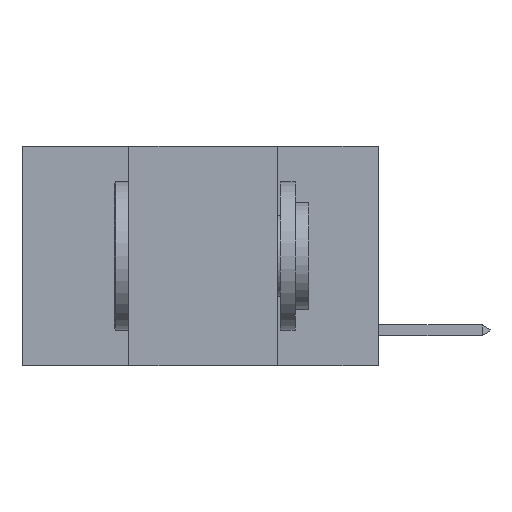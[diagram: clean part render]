
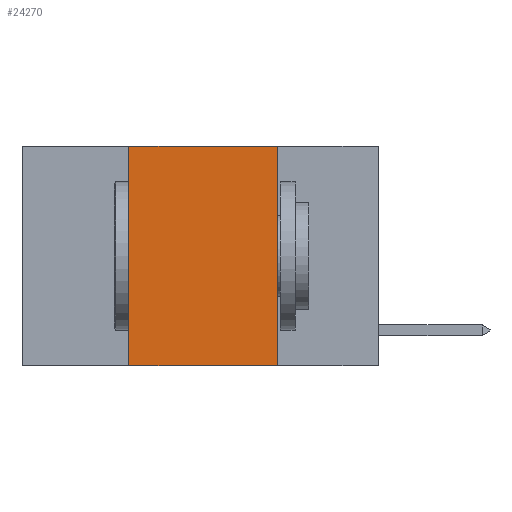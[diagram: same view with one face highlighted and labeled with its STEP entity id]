
A CAD part, left-side view. The second image highlights one B-rep face of the part: STEP entity #24270.
In plain terms, the highlighted planar face has unit normal (-1, 0, 0).
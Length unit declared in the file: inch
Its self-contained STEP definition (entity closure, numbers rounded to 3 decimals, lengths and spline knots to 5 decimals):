
#170 = VECTOR ( 'NONE', #6098, 39.37008 ) ;
#494 = CARTESIAN_POINT ( 'NONE',  ( 0., 0.6, -0.37 ) ) ;
#537 = CARTESIAN_POINT ( 'NONE',  ( 0., 0.17, 0. ) ) ;
#1987 = DIRECTION ( 'NONE',  ( 1., 0., 0. ) ) ;
#2292 = VECTOR ( 'NONE', #11630, 39.37008 ) ;
#3111 = ORIENTED_EDGE ( 'NONE', *, *, #17159, .F. ) ;
#4316 = ORIENTED_EDGE ( 'NONE', *, *, #19975, .T. ) ;
#4375 = DIRECTION ( 'NONE',  ( 0., 0., -1. ) ) ;
#5484 = AXIS2_PLACEMENT_3D ( 'NONE', #13439, #1987, #15353 ) ;
#5753 = PLANE ( 'NONE',  #5484 ) ;
#5839 = CARTESIAN_POINT ( 'NONE',  ( 0., 0.42, -0.37 ) ) ;
#6098 = DIRECTION ( 'NONE',  ( 0., 0., 1. ) ) ;
#6140 = CARTESIAN_POINT ( 'NONE',  ( 0., 0.17, -0.37 ) ) ;
#7251 = VERTEX_POINT ( 'NONE', #14531 ) ;
#7388 = LINE ( 'NONE', #17176, #2292 ) ;
#8005 = CARTESIAN_POINT ( 'NONE',  ( 0., 0.42, 0. ) ) ;
#8084 = DIRECTION ( 'NONE',  ( 0., -1., 0. ) ) ;
#8748 = EDGE_CURVE ( 'NONE', #18303, #7251, #7388, .T. ) ;
#8791 = ORIENTED_EDGE ( 'NONE', *, *, #8748, .F. ) ;
#8837 = LINE ( 'NONE', #537, #13332 ) ;
#9439 = VERTEX_POINT ( 'NONE', #5839 ) ;
#9507 = EDGE_CURVE ( 'NONE', #9439, #18303, #10306, .T. ) ;
#9645 = CARTESIAN_POINT ( 'NONE',  ( 0., 0.42, 0. ) ) ;
#9782 = VECTOR ( 'NONE', #8084, 39.37008 ) ;
#10306 = LINE ( 'NONE', #8005, #170 ) ;
#11630 = DIRECTION ( 'NONE',  ( 0., -1., 0. ) ) ;
#13332 = VECTOR ( 'NONE', #4375, 39.37008 ) ;
#13439 = CARTESIAN_POINT ( 'NONE',  ( 0., 0.6, 0. ) ) ;
#13884 = ORIENTED_EDGE ( 'NONE', *, *, #9507, .F. ) ;
#14038 = VERTEX_POINT ( 'NONE', #6140 ) ;
#14531 = CARTESIAN_POINT ( 'NONE',  ( 0., 0.17, 0. ) ) ;
#14981 = EDGE_LOOP ( 'NONE', ( #3111, #8791, #13884, #4316 ) ) ;
#15353 = DIRECTION ( 'NONE',  ( 0., 0., -1. ) ) ;
#17159 = EDGE_CURVE ( 'NONE', #7251, #14038, #8837, .T. ) ;
#17176 = CARTESIAN_POINT ( 'NONE',  ( 0., 0.6, 0. ) ) ;
#18303 = VERTEX_POINT ( 'NONE', #9645 ) ;
#18769 = FACE_OUTER_BOUND ( 'NONE', #14981, .T. ) ;
#19975 = EDGE_CURVE ( 'NONE', #9439, #14038, #23076, .T. ) ;
#23076 = LINE ( 'NONE', #494, #9782 ) ;
#24270 = ADVANCED_FACE ( 'NONE', ( #18769 ), #5753, .F. ) ;
